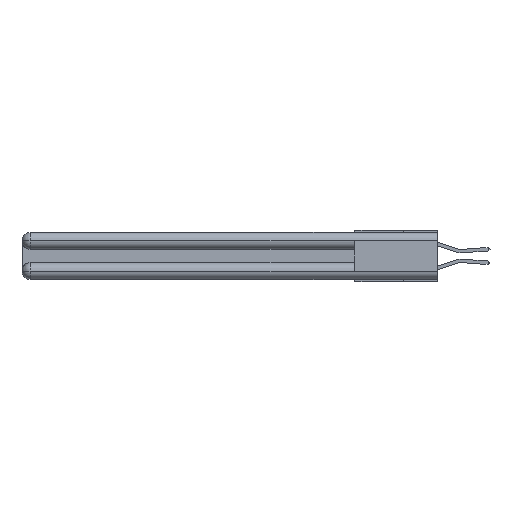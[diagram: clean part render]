
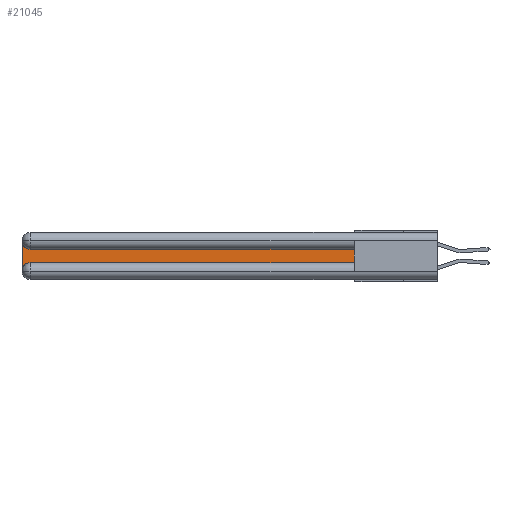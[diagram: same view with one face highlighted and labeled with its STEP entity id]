
A CAD part, left-side view. The second image highlights one B-rep face of the part: STEP entity #21045.
In plain terms, the highlighted planar face has unit normal (-1, 0, 0).
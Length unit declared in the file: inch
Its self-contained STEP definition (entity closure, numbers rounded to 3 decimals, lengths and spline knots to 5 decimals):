
#458 = CARTESIAN_POINT ( 'NONE',  ( 0.075, 3., -0.1225 ) ) ;
#483 = CARTESIAN_POINT ( 'NONE',  ( 0.075, 0.6, -0.2175 ) ) ;
#2425 = AXIS2_PLACEMENT_3D ( 'NONE', #458, #13221, #15736 ) ;
#4678 = VERTEX_POINT ( 'NONE', #10758 ) ;
#6230 = DIRECTION ( 'NONE',  ( 0., 0., -1. ) ) ;
#6257 = CARTESIAN_POINT ( 'NONE',  ( 0.075, 2.94, -0.2175 ) ) ;
#6770 = DIRECTION ( 'NONE',  ( 0., 0., 1. ) ) ;
#7362 = VERTEX_POINT ( 'NONE', #27755 ) ;
#7769 = EDGE_LOOP ( 'NONE', ( #26556, #25090, #7975, #8630, #17150, #19438 ) ) ;
#7975 = ORIENTED_EDGE ( 'NONE', *, *, #11765, .T. ) ;
#8210 = VERTEX_POINT ( 'NONE', #6257 ) ;
#8630 = ORIENTED_EDGE ( 'NONE', *, *, #18175, .T. ) ;
#10758 = CARTESIAN_POINT ( 'NONE',  ( 0.075, 3., -0.0625 ) ) ;
#11765 = EDGE_CURVE ( 'NONE', #4678, #21073, #27855, .T. ) ;
#11833 = DIRECTION ( 'NONE',  ( 1., 0., 0. ) ) ;
#12440 = EDGE_CURVE ( 'NONE', #16463, #4678, #21440, .T. ) ;
#12598 = CARTESIAN_POINT ( 'NONE',  ( 0.075, 0.6, -0.1225 ) ) ;
#13221 = DIRECTION ( 'NONE',  ( 1., 0., 0. ) ) ;
#13327 = VECTOR ( 'NONE', #17314, 39.37008 ) ;
#15302 = FACE_OUTER_BOUND ( 'NONE', #7769, .T. ) ;
#15736 = DIRECTION ( 'NONE',  ( 0., 0., -1. ) ) ;
#16138 = EDGE_CURVE ( 'NONE', #8210, #22196, #23502, .T. ) ;
#16401 = DIRECTION ( 'NONE',  ( 1., 0., 0. ) ) ;
#16463 = VERTEX_POINT ( 'NONE', #19950 ) ;
#16689 = VECTOR ( 'NONE', #6230, 39.37008 ) ;
#16695 = CARTESIAN_POINT ( 'NONE',  ( 0.075, 3., -0.2775 ) ) ;
#16701 = AXIS2_PLACEMENT_3D ( 'NONE', #20637, #11833, #24519 ) ;
#16759 = DIRECTION ( 'NONE',  ( 0., -1., 0. ) ) ;
#17034 = CARTESIAN_POINT ( 'NONE',  ( 0.075, 0.6, -0.2175 ) ) ;
#17150 = ORIENTED_EDGE ( 'NONE', *, *, #16138, .T. ) ;
#17314 = DIRECTION ( 'NONE',  ( 0., 1., 0. ) ) ;
#18175 = EDGE_CURVE ( 'NONE', #21073, #8210, #18591, .T. ) ;
#18591 = CIRCLE ( 'NONE', #16701, 0.06 ) ;
#18740 = LINE ( 'NONE', #483, #25822 ) ;
#19438 = ORIENTED_EDGE ( 'NONE', *, *, #21443, .T. ) ;
#19950 = CARTESIAN_POINT ( 'NONE',  ( 0.075, 2.94, -0.1225 ) ) ;
#20637 = CARTESIAN_POINT ( 'NONE',  ( 0.075, 2.94, -0.2775 ) ) ;
#20846 = LINE ( 'NONE', #12598, #13327 ) ;
#21045 = ADVANCED_FACE ( 'NONE', ( #15302 ), #26264, .F. ) ;
#21073 = VERTEX_POINT ( 'NONE', #16695 ) ;
#21440 = CIRCLE ( 'NONE', #27299, 0.06 ) ;
#21443 = EDGE_CURVE ( 'NONE', #22196, #7362, #18740, .T. ) ;
#22138 = VECTOR ( 'NONE', #16759, 39.37008 ) ;
#22196 = VERTEX_POINT ( 'NONE', #26770 ) ;
#23502 = LINE ( 'NONE', #17034, #22138 ) ;
#23511 = CARTESIAN_POINT ( 'NONE',  ( 0.075, 3., -0.2175 ) ) ;
#24519 = DIRECTION ( 'NONE',  ( 0., 0., -1. ) ) ;
#25009 = CARTESIAN_POINT ( 'NONE',  ( 0.075, 2.94, -0.0625 ) ) ;
#25090 = ORIENTED_EDGE ( 'NONE', *, *, #12440, .T. ) ;
#25295 = EDGE_CURVE ( 'NONE', #7362, #16463, #20846, .T. ) ;
#25392 = DIRECTION ( 'NONE',  ( 0., 0., -1. ) ) ;
#25822 = VECTOR ( 'NONE', #6770, 39.37008 ) ;
#26264 = PLANE ( 'NONE',  #2425 ) ;
#26556 = ORIENTED_EDGE ( 'NONE', *, *, #25295, .T. ) ;
#26770 = CARTESIAN_POINT ( 'NONE',  ( 0.075, 0.6, -0.2175 ) ) ;
#27299 = AXIS2_PLACEMENT_3D ( 'NONE', #25009, #16401, #25392 ) ;
#27755 = CARTESIAN_POINT ( 'NONE',  ( 0.075, 0.6, -0.1225 ) ) ;
#27855 = LINE ( 'NONE', #23511, #16689 ) ;
